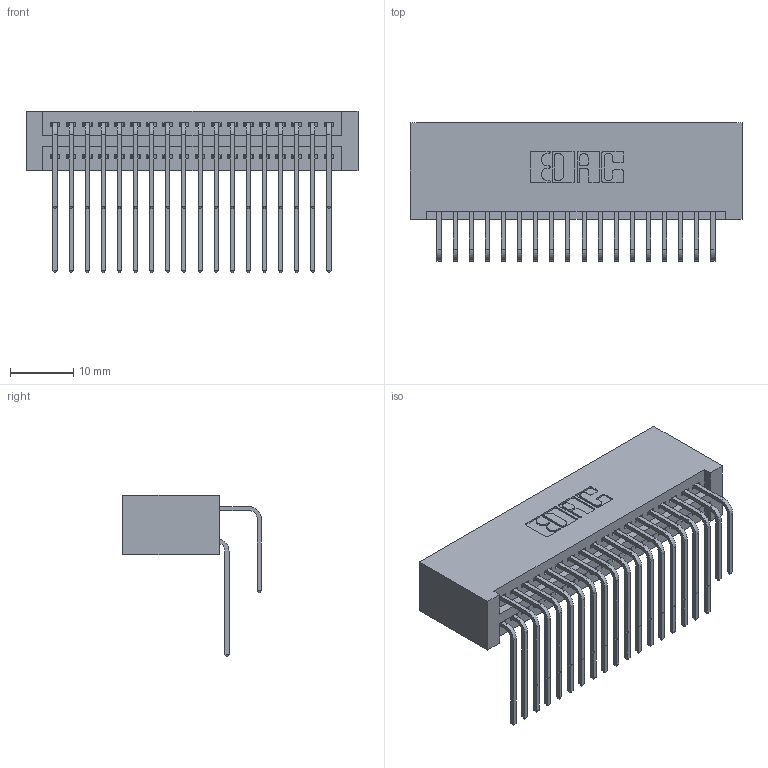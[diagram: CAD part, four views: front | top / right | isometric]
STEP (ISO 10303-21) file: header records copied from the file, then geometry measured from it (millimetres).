
FILE_DESCRIPTION (( 'STEP AP203' ), '1' );
FILE_NAME ('395-036-558-201.STEP', '2019-10-18T02:54:57', ( '' ), ( '' ), 'SwSTEP 2.0', 'SolidWorks 2016', '' );
FILE_SCHEMA (( 'CONFIG_CONTROL_DESIGN' ));
Length unit declared in the file: inch
Products named in the file (4): 395-036-558-201; 345 Part_No Mounting Lugs; 345-292-001_558 559 Tail - 1; 345-292-001_558 Tail - 2
Assembly tree (37 placements, depth 2):
  395-036-558-201
    345 Part_No Mounting Lugs
    345-292-001_558 559 Tail - 1  x18
    345-292-001_558 Tail - 2  x18
Bounding box: 52.32 x 21.83 x 25.53 mm (x, y, z)
Volume: 5683.6 mm3; surface area: 9216.3 mm2
Topology: 37 solids, 37 shells, 1990 faces, 5897 edges, 3882 vertices
Faces by surface type: plane 1336, cylinder 654
Entity records: 18729 total; most frequent: CARTESIAN_POINT 3207, ORIENTED_EDGE 3090, DIRECTION 2825, EDGE_CURVE 1545, LINE 1309, VECTOR 1309, VERTEX_POINT 1026, AXIS2_PLACEMENT_3D 758
